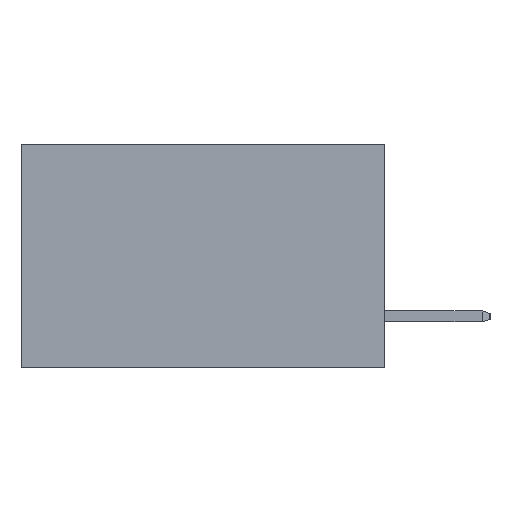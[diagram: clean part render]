
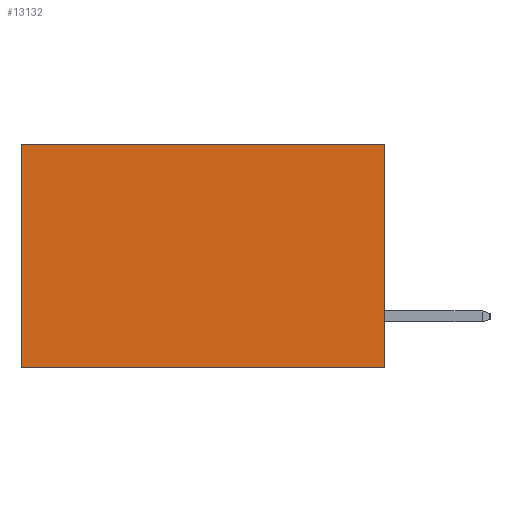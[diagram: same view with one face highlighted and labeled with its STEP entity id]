
A CAD part, left-side view. The second image highlights one B-rep face of the part: STEP entity #13132.
In plain terms, the highlighted planar face has unit normal (-1, 0, 0).
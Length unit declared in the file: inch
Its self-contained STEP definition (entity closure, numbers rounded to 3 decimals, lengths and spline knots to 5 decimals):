
#435 = EDGE_CURVE ( 'NONE', #3052, #4680, #7232, .T. ) ;
#598 = ORIENTED_EDGE ( 'NONE', *, *, #435, .T. ) ;
#1187 = VECTOR ( 'NONE', #15406, 39.37008 ) ;
#1479 = DIRECTION ( 'NONE',  ( 0., 0., -1. ) ) ;
#1994 = ORIENTED_EDGE ( 'NONE', *, *, #11500, .F. ) ;
#2245 = EDGE_CURVE ( 'NONE', #7564, #10246, #11720, .T. ) ;
#3052 = VERTEX_POINT ( 'NONE', #7202 ) ;
#3110 = EDGE_CURVE ( 'NONE', #7564, #3052, #4592, .T. ) ;
#3556 = AXIS2_PLACEMENT_3D ( 'NONE', #12571, #9088, #1479 ) ;
#4580 = CARTESIAN_POINT ( 'NONE',  ( 0.2615, 0.6, -0.37 ) ) ;
#4592 = LINE ( 'NONE', #8656, #15768 ) ;
#4680 = VERTEX_POINT ( 'NONE', #4580 ) ;
#5300 = CARTESIAN_POINT ( 'NONE',  ( 0.2615, 0., 0. ) ) ;
#5776 = EDGE_LOOP ( 'NONE', ( #598, #1994, #8001, #14147 ) ) ;
#6795 = DIRECTION ( 'NONE',  ( 0., 0., -1. ) ) ;
#6879 = CARTESIAN_POINT ( 'NONE',  ( 0.2615, 0.6, -0.37 ) ) ;
#7152 = CARTESIAN_POINT ( 'NONE',  ( 0.2615, 0., -0.37 ) ) ;
#7202 = CARTESIAN_POINT ( 'NONE',  ( 0.2615, 0.6, 0. ) ) ;
#7232 = LINE ( 'NONE', #6879, #9774 ) ;
#7564 = VERTEX_POINT ( 'NONE', #5300 ) ;
#8001 = ORIENTED_EDGE ( 'NONE', *, *, #2245, .F. ) ;
#8465 = DIRECTION ( 'NONE',  ( 0., 1., 0. ) ) ;
#8496 = FACE_OUTER_BOUND ( 'NONE', #5776, .T. ) ;
#8656 = CARTESIAN_POINT ( 'NONE',  ( 0.2615, 0., 0. ) ) ;
#8787 = CARTESIAN_POINT ( 'NONE',  ( 0.2615, 0., -0.37 ) ) ;
#9088 = DIRECTION ( 'NONE',  ( 1., 0., 0. ) ) ;
#9774 = VECTOR ( 'NONE', #6795, 39.37008 ) ;
#10246 = VERTEX_POINT ( 'NONE', #8787 ) ;
#10825 = LINE ( 'NONE', #7152, #1187 ) ;
#11500 = EDGE_CURVE ( 'NONE', #10246, #4680, #10825, .T. ) ;
#11720 = LINE ( 'NONE', #13947, #14777 ) ;
#12571 = CARTESIAN_POINT ( 'NONE',  ( 0.2615, 0., -0.37 ) ) ;
#13132 = ADVANCED_FACE ( 'NONE', ( #8496 ), #14833, .F. ) ;
#13947 = CARTESIAN_POINT ( 'NONE',  ( 0.2615, 0., -0.37 ) ) ;
#14147 = ORIENTED_EDGE ( 'NONE', *, *, #3110, .T. ) ;
#14777 = VECTOR ( 'NONE', #15307, 39.37008 ) ;
#14833 = PLANE ( 'NONE',  #3556 ) ;
#15307 = DIRECTION ( 'NONE',  ( 0., 0., -1. ) ) ;
#15406 = DIRECTION ( 'NONE',  ( 0., 1., 0. ) ) ;
#15768 = VECTOR ( 'NONE', #8465, 39.37008 ) ;
